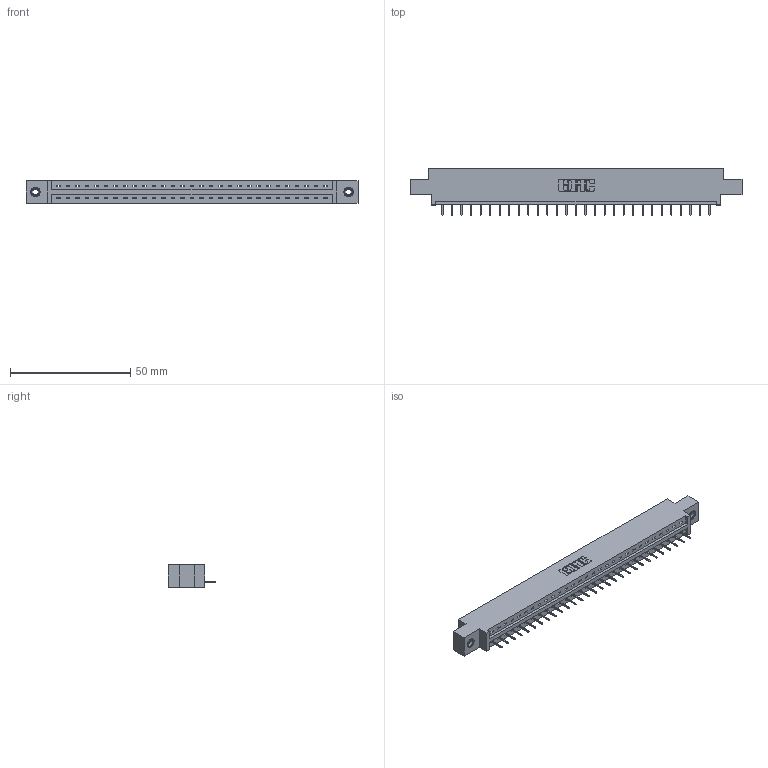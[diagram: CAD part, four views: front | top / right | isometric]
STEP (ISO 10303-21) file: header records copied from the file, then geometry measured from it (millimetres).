
FILE_DESCRIPTION (( 'STEP AP203' ), '1' );
FILE_NAME ('387-029-524-608.STEP', '2019-10-03T17:05:37', ( '' ), ( '' ), 'SwSTEP 2.0', 'SolidWorks 2016', '' );
FILE_SCHEMA (( 'CONFIG_CONTROL_DESIGN' ));
Length unit declared in the file: inch
Products named in the file (4): 345-292-001_345-293-124; 345-250-001_345-250-003-102; 337 Part_0.170 Offset - 0.156 Dia-TI; 387-029-524-608
Assembly tree (32 placements, depth 2):
  387-029-524-608
    337 Part_0.170 Offset - 0.156 Dia-TI
    345-292-001_345-293-124  x29
    345-250-001_345-250-003-102  x2
Bounding box: 137.92 x 19.69 x 9.4 mm (x, y, z)
Volume: 13933.4 mm3; surface area: 14049.2 mm2
Topology: 32 solids, 32 shells, 2092 faces, 6027 edges, 3894 vertices
Faces by surface type: plane 1614, cylinder 462, cone 12, torus 4
Entity records: 24630 total; most frequent: CARTESIAN_POINT 4268, ORIENTED_EDGE 4226, DIRECTION 3653, EDGE_CURVE 2113, VECTOR 1969, LINE 1969, VERTEX_POINT 1400, AXIS2_PLACEMENT_3D 842
